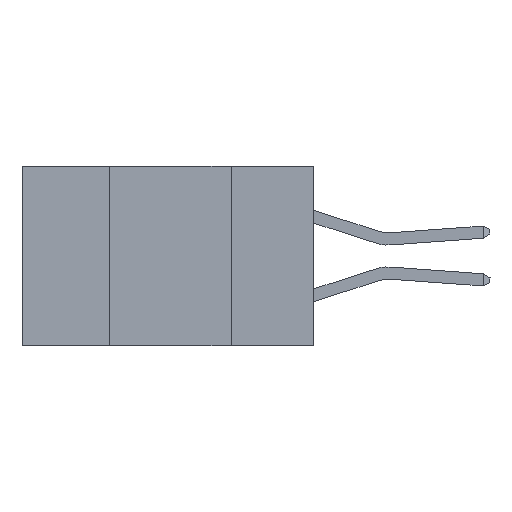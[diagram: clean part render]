
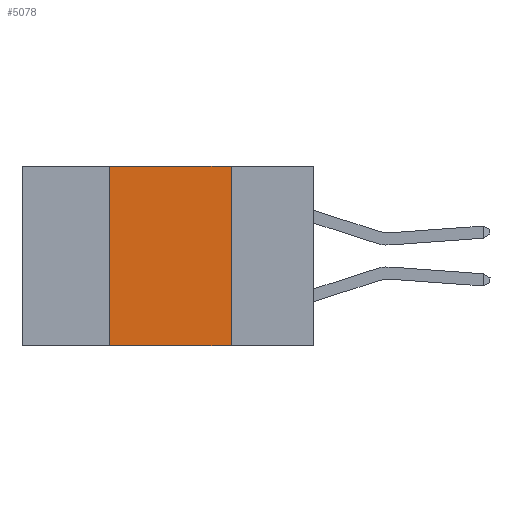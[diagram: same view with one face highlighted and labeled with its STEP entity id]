
A CAD part, left-side view. The second image highlights one B-rep face of the part: STEP entity #5078.
In plain terms, the highlighted planar face has unit normal (-1, 0, 0).
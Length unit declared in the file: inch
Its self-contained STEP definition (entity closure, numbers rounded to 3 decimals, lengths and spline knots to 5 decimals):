
#214 = VECTOR ( 'NONE', #4437, 39.37008 ) ;
#354 = CARTESIAN_POINT ( 'NONE',  ( 0., 0.42, 0. ) ) ;
#449 = CARTESIAN_POINT ( 'NONE',  ( 0., 0.17, 0. ) ) ;
#1283 = CARTESIAN_POINT ( 'NONE',  ( 0., 0.42, -0.37 ) ) ;
#1893 = LINE ( 'NONE', #10817, #5015 ) ;
#2665 = LINE ( 'NONE', #8952, #214 ) ;
#3540 = ORIENTED_EDGE ( 'NONE', *, *, #5490, .F. ) ;
#3738 = FACE_OUTER_BOUND ( 'NONE', #9139, .T. ) ;
#3823 = VECTOR ( 'NONE', #11330, 39.37008 ) ;
#4192 = EDGE_CURVE ( 'NONE', #8299, #11680, #2665, .T. ) ;
#4214 = CARTESIAN_POINT ( 'NONE',  ( 0., 0.6, 0. ) ) ;
#4437 = DIRECTION ( 'NONE',  ( 0., -1., 0. ) ) ;
#4861 = PLANE ( 'NONE',  #10797 ) ;
#5015 = VECTOR ( 'NONE', #8177, 39.37008 ) ;
#5078 = ADVANCED_FACE ( 'NONE', ( #3738 ), #4861, .F. ) ;
#5104 = VERTEX_POINT ( 'NONE', #354 ) ;
#5136 = DIRECTION ( 'NONE',  ( 0., -1., 0. ) ) ;
#5352 = CARTESIAN_POINT ( 'NONE',  ( 0., 0.17, -0.37 ) ) ;
#5490 = EDGE_CURVE ( 'NONE', #8299, #5104, #1893, .T. ) ;
#5661 = CARTESIAN_POINT ( 'NONE',  ( 0., 0.17, 0. ) ) ;
#5713 = CARTESIAN_POINT ( 'NONE',  ( 0., 0.6, 0. ) ) ;
#5793 = DIRECTION ( 'NONE',  ( 0., 0., -1. ) ) ;
#6849 = VECTOR ( 'NONE', #5136, 39.37008 ) ;
#7513 = LINE ( 'NONE', #449, #3823 ) ;
#7815 = EDGE_CURVE ( 'NONE', #8844, #11680, #7513, .T. ) ;
#7965 = LINE ( 'NONE', #4214, #6849 ) ;
#8177 = DIRECTION ( 'NONE',  ( 0., 0., 1. ) ) ;
#8299 = VERTEX_POINT ( 'NONE', #1283 ) ;
#8322 = ORIENTED_EDGE ( 'NONE', *, *, #4192, .T. ) ;
#8379 = DIRECTION ( 'NONE',  ( 1., 0., 0. ) ) ;
#8633 = ORIENTED_EDGE ( 'NONE', *, *, #11153, .F. ) ;
#8844 = VERTEX_POINT ( 'NONE', #5661 ) ;
#8952 = CARTESIAN_POINT ( 'NONE',  ( 0., 0.6, -0.37 ) ) ;
#9139 = EDGE_LOOP ( 'NONE', ( #9230, #8633, #3540, #8322 ) ) ;
#9230 = ORIENTED_EDGE ( 'NONE', *, *, #7815, .F. ) ;
#10797 = AXIS2_PLACEMENT_3D ( 'NONE', #5713, #8379, #5793 ) ;
#10817 = CARTESIAN_POINT ( 'NONE',  ( 0., 0.42, 0. ) ) ;
#11153 = EDGE_CURVE ( 'NONE', #5104, #8844, #7965, .T. ) ;
#11330 = DIRECTION ( 'NONE',  ( 0., 0., -1. ) ) ;
#11680 = VERTEX_POINT ( 'NONE', #5352 ) ;
